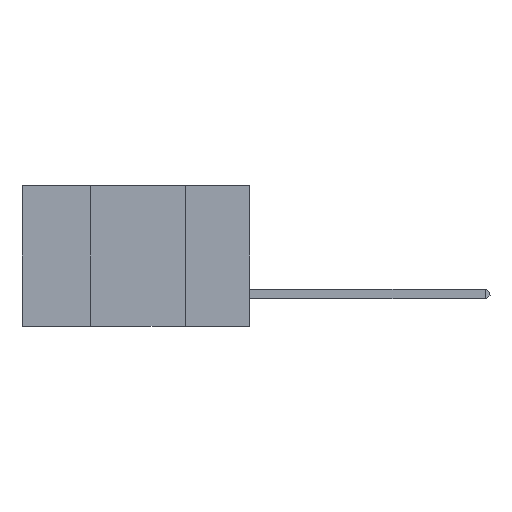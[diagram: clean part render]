
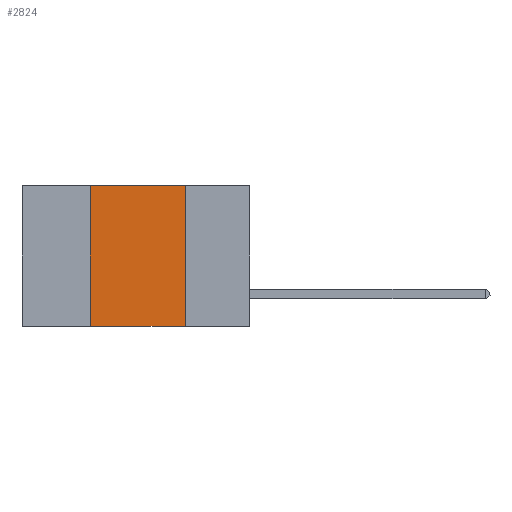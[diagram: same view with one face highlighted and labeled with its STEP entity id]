
A CAD part, left-side view. The second image highlights one B-rep face of the part: STEP entity #2824.
In plain terms, the highlighted planar face has unit normal (-1, 0, 0).
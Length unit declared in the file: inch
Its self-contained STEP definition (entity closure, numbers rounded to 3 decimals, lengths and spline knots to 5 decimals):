
#80 = EDGE_CURVE ( 'NONE', #2883, #9427, #3337, .T. ) ;
#250 = VECTOR ( 'NONE', #13391, 39.37008 ) ;
#289 = DIRECTION ( 'NONE',  ( 1., 0., 0. ) ) ;
#673 = DIRECTION ( 'NONE',  ( 0., 0., 1. ) ) ;
#847 = EDGE_LOOP ( 'NONE', ( #7714, #16303, #12609, #2603 ) ) ;
#1158 = CARTESIAN_POINT ( 'NONE',  ( 0., 0.17, -0.37 ) ) ;
#1475 = LINE ( 'NONE', #3749, #250 ) ;
#1735 = CARTESIAN_POINT ( 'NONE',  ( 0., 0.17, 0. ) ) ;
#1930 = VERTEX_POINT ( 'NONE', #5890 ) ;
#2603 = ORIENTED_EDGE ( 'NONE', *, *, #10729, .T. ) ;
#2722 = DIRECTION ( 'NONE',  ( 0., 0., -1. ) ) ;
#2824 = ADVANCED_FACE ( 'NONE', ( #16559 ), #11931, .F. ) ;
#2883 = VERTEX_POINT ( 'NONE', #4115 ) ;
#3337 = LINE ( 'NONE', #13014, #12937 ) ;
#3749 = CARTESIAN_POINT ( 'NONE',  ( 0., 0.17, 0. ) ) ;
#3795 = AXIS2_PLACEMENT_3D ( 'NONE', #13226, #289, #2722 ) ;
#4115 = CARTESIAN_POINT ( 'NONE',  ( 0., 0.42, 0. ) ) ;
#4559 = CARTESIAN_POINT ( 'NONE',  ( 0., 0.42, 0. ) ) ;
#5890 = CARTESIAN_POINT ( 'NONE',  ( 0., 0.42, -0.37 ) ) ;
#6526 = EDGE_CURVE ( 'NONE', #1930, #2883, #12348, .T. ) ;
#7714 = ORIENTED_EDGE ( 'NONE', *, *, #14014, .F. ) ;
#7889 = VECTOR ( 'NONE', #673, 39.37008 ) ;
#9427 = VERTEX_POINT ( 'NONE', #1735 ) ;
#9503 = CARTESIAN_POINT ( 'NONE',  ( 0., 0.6, -0.37 ) ) ;
#10729 = EDGE_CURVE ( 'NONE', #1930, #15550, #14559, .T. ) ;
#11087 = VECTOR ( 'NONE', #14058, 39.37008 ) ;
#11781 = DIRECTION ( 'NONE',  ( 0., -1., 0. ) ) ;
#11931 = PLANE ( 'NONE',  #3795 ) ;
#12348 = LINE ( 'NONE', #4559, #7889 ) ;
#12609 = ORIENTED_EDGE ( 'NONE', *, *, #6526, .F. ) ;
#12937 = VECTOR ( 'NONE', #11781, 39.37008 ) ;
#13014 = CARTESIAN_POINT ( 'NONE',  ( 0., 0.6, 0. ) ) ;
#13226 = CARTESIAN_POINT ( 'NONE',  ( 0., 0.6, 0. ) ) ;
#13391 = DIRECTION ( 'NONE',  ( 0., 0., -1. ) ) ;
#14014 = EDGE_CURVE ( 'NONE', #9427, #15550, #1475, .T. ) ;
#14058 = DIRECTION ( 'NONE',  ( 0., -1., 0. ) ) ;
#14559 = LINE ( 'NONE', #9503, #11087 ) ;
#15550 = VERTEX_POINT ( 'NONE', #1158 ) ;
#16303 = ORIENTED_EDGE ( 'NONE', *, *, #80, .F. ) ;
#16559 = FACE_OUTER_BOUND ( 'NONE', #847, .T. ) ;
